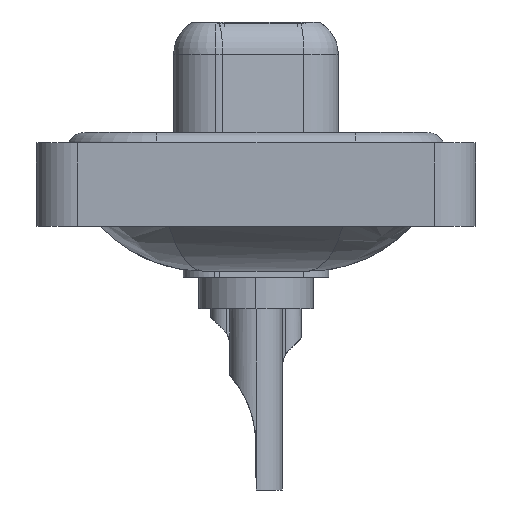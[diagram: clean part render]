
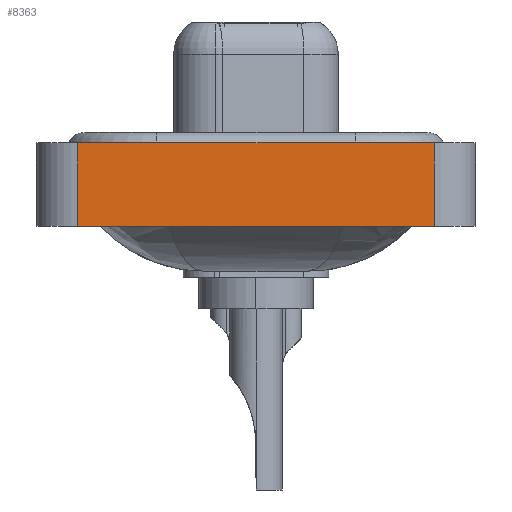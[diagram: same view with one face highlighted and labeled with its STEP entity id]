
A CAD part, left-side view. The second image highlights one B-rep face of the part: STEP entity #8363.
In plain terms, the highlighted planar face has unit normal (-1, 0, 0).
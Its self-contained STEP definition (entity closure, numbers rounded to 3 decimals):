
#353 = CARTESIAN_POINT ( 'NONE',  ( -7.35, 8.55, -3.6 ) ) ;
#585 = FACE_OUTER_BOUND ( 'NONE', #17224, .T. ) ;
#1968 = DIRECTION ( 'NONE',  ( -1., 0., 0. ) ) ;
#2319 = DIRECTION ( 'NONE',  ( 0., 0., 1. ) ) ;
#2514 = EDGE_CURVE ( 'NONE', #22471, #18619, #14521, .T. ) ;
#2859 = VECTOR ( 'NONE', #2319, 1000. ) ;
#2868 = LINE ( 'NONE', #9673, #3488 ) ;
#3066 = ORIENTED_EDGE ( 'NONE', *, *, #3178, .F. ) ;
#3178 = EDGE_CURVE ( 'NONE', #18619, #20784, #2868, .T. ) ;
#3488 = VECTOR ( 'NONE', #20314, 1000. ) ;
#5255 = CARTESIAN_POINT ( 'NONE',  ( -7.35, -8.55, -3.6 ) ) ;
#7305 = VECTOR ( 'NONE', #11966, 1000. ) ;
#7405 = CARTESIAN_POINT ( 'NONE',  ( -7.35, 8.55, 0.4 ) ) ;
#8363 = ADVANCED_FACE ( 'NONE', ( #585 ), #12743, .T. ) ;
#8485 = ORIENTED_EDGE ( 'NONE', *, *, #19540, .T. ) ;
#9000 = VERTEX_POINT ( 'NONE', #16583 ) ;
#9509 = EDGE_CURVE ( 'NONE', #22471, #9000, #15953, .T. ) ;
#9673 = CARTESIAN_POINT ( 'NONE',  ( -7.35, -8.55, 0.4 ) ) ;
#9876 = AXIS2_PLACEMENT_3D ( 'NONE', #21883, #1968, #14753 ) ;
#11653 = CARTESIAN_POINT ( 'NONE',  ( -7.35, -8.55, 0.4 ) ) ;
#11966 = DIRECTION ( 'NONE',  ( 0., -1., 0. ) ) ;
#12280 = LINE ( 'NONE', #19397, #19155 ) ;
#12743 = PLANE ( 'NONE',  #9876 ) ;
#12879 = CARTESIAN_POINT ( 'NONE',  ( -7.35, 8.55, -3.6 ) ) ;
#12976 = ORIENTED_EDGE ( 'NONE', *, *, #9509, .T. ) ;
#14521 = LINE ( 'NONE', #12879, #2859 ) ;
#14753 = DIRECTION ( 'NONE',  ( 0., 0., 1. ) ) ;
#15953 = LINE ( 'NONE', #5255, #7305 ) ;
#16352 = ORIENTED_EDGE ( 'NONE', *, *, #2514, .F. ) ;
#16583 = CARTESIAN_POINT ( 'NONE',  ( -7.35, -8.55, -3.6 ) ) ;
#17224 = EDGE_LOOP ( 'NONE', ( #8485, #3066, #16352, #12976 ) ) ;
#17890 = DIRECTION ( 'NONE',  ( 0., 0., 1. ) ) ;
#18619 = VERTEX_POINT ( 'NONE', #7405 ) ;
#19155 = VECTOR ( 'NONE', #17890, 1000. ) ;
#19397 = CARTESIAN_POINT ( 'NONE',  ( -7.35, -8.55, -3.6 ) ) ;
#19540 = EDGE_CURVE ( 'NONE', #9000, #20784, #12280, .T. ) ;
#20314 = DIRECTION ( 'NONE',  ( 0., -1., 0. ) ) ;
#20784 = VERTEX_POINT ( 'NONE', #11653 ) ;
#21883 = CARTESIAN_POINT ( 'NONE',  ( -7.35, -8.55, -3.6 ) ) ;
#22471 = VERTEX_POINT ( 'NONE', #353 ) ;
